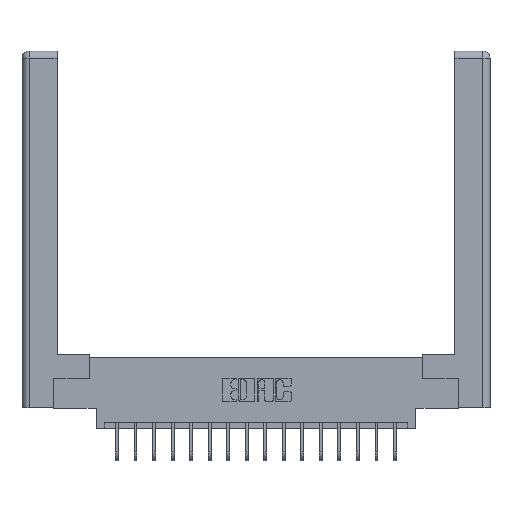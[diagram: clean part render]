
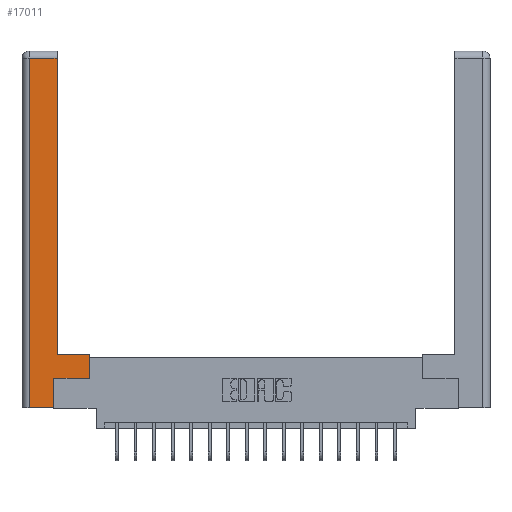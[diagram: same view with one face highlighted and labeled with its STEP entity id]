
A CAD part, top view. The second image highlights one B-rep face of the part: STEP entity #17011.
In plain terms, the highlighted planar face has unit normal (0, 0, 1).
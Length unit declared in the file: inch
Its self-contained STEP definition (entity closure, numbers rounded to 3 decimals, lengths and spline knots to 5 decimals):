
#185 = CARTESIAN_POINT ( 'NONE',  ( 0.265, 0.245, 0. ) ) ;
#501 = EDGE_CURVE ( 'NONE', #12441, #10015, #13441, .T. ) ;
#555 = VERTEX_POINT ( 'NONE', #2148 ) ;
#825 = LINE ( 'NONE', #7558, #19997 ) ;
#933 = CARTESIAN_POINT ( 'NONE',  ( 0.265, 0.245, 0. ) ) ;
#1471 = LINE ( 'NONE', #16307, #1960 ) ;
#1728 = CARTESIAN_POINT ( 'NONE',  ( 0.565, 0.245, 0. ) ) ;
#1729 = ORIENTED_EDGE ( 'NONE', *, *, #9157, .T. ) ;
#1960 = VECTOR ( 'NONE', #11657, 39.37008 ) ;
#2148 = CARTESIAN_POINT ( 'NONE',  ( 0.565, 0.245, 0. ) ) ;
#2303 = EDGE_LOOP ( 'NONE', ( #12869, #15334, #15696, #9023, #11551, #5707, #1729, #14557 ) ) ;
#2415 = PLANE ( 'NONE',  #19945 ) ;
#2545 = VECTOR ( 'NONE', #11239, 39.37008 ) ;
#3287 = CARTESIAN_POINT ( 'NONE',  ( 0.0615, 2.94, 0. ) ) ;
#4849 = DIRECTION ( 'NONE',  ( -1., 0., 0. ) ) ;
#4950 = CARTESIAN_POINT ( 'NONE',  ( 0.295, 2.94, 0. ) ) ;
#5299 = CARTESIAN_POINT ( 'NONE',  ( 0., 0., 0. ) ) ;
#5707 = ORIENTED_EDGE ( 'NONE', *, *, #6913, .T. ) ;
#6329 = EDGE_CURVE ( 'NONE', #10642, #17153, #825, .T. ) ;
#6685 = DIRECTION ( 'NONE',  ( -1., 0., 0. ) ) ;
#6752 = LINE ( 'NONE', #1728, #2545 ) ;
#6913 = EDGE_CURVE ( 'NONE', #12769, #555, #6752, .T. ) ;
#7241 = DIRECTION ( 'NONE',  ( -1., 0., 0. ) ) ;
#7310 = LINE ( 'NONE', #19363, #11980 ) ;
#7325 = VECTOR ( 'NONE', #4849, 39.37008 ) ;
#7428 = EDGE_CURVE ( 'NONE', #17153, #12769, #11880, .T. ) ;
#7558 = CARTESIAN_POINT ( 'NONE',  ( 0.265, 0., 0. ) ) ;
#8704 = VECTOR ( 'NONE', #11945, 39.37008 ) ;
#8774 = DIRECTION ( 'NONE',  ( 0., 0., -1. ) ) ;
#8837 = EDGE_CURVE ( 'NONE', #10015, #18423, #1471, .T. ) ;
#9023 = ORIENTED_EDGE ( 'NONE', *, *, #6329, .T. ) ;
#9157 = EDGE_CURVE ( 'NONE', #555, #12441, #19403, .T. ) ;
#9784 = VERTEX_POINT ( 'NONE', #3287 ) ;
#9792 = EDGE_CURVE ( 'NONE', #18423, #9784, #9849, .T. ) ;
#9849 = LINE ( 'NONE', #18941, #7325 ) ;
#10015 = VERTEX_POINT ( 'NONE', #18002 ) ;
#10030 = CARTESIAN_POINT ( 'NONE',  ( 0.0615, 0., 0. ) ) ;
#10642 = VERTEX_POINT ( 'NONE', #10030 ) ;
#10835 = FACE_OUTER_BOUND ( 'NONE', #2303, .T. ) ;
#11089 = VECTOR ( 'NONE', #17336, 39.37008 ) ;
#11239 = DIRECTION ( 'NONE',  ( 1., 0., 0. ) ) ;
#11551 = ORIENTED_EDGE ( 'NONE', *, *, #7428, .T. ) ;
#11657 = DIRECTION ( 'NONE',  ( 0., 1., 0. ) ) ;
#11724 = EDGE_CURVE ( 'NONE', #9784, #10642, #7310, .T. ) ;
#11880 = LINE ( 'NONE', #933, #8704 ) ;
#11945 = DIRECTION ( 'NONE',  ( 0., 1., 0. ) ) ;
#11976 = VECTOR ( 'NONE', #6685, 39.37008 ) ;
#11980 = VECTOR ( 'NONE', #14733, 39.37008 ) ;
#12441 = VERTEX_POINT ( 'NONE', #13659 ) ;
#12769 = VERTEX_POINT ( 'NONE', #185 ) ;
#12869 = ORIENTED_EDGE ( 'NONE', *, *, #8837, .T. ) ;
#13441 = LINE ( 'NONE', #17613, #11976 ) ;
#13659 = CARTESIAN_POINT ( 'NONE',  ( 0.565, 0.45, 0. ) ) ;
#14557 = ORIENTED_EDGE ( 'NONE', *, *, #501, .T. ) ;
#14733 = DIRECTION ( 'NONE',  ( 0., -1., 0. ) ) ;
#15334 = ORIENTED_EDGE ( 'NONE', *, *, #9792, .T. ) ;
#15696 = ORIENTED_EDGE ( 'NONE', *, *, #11724, .T. ) ;
#16307 = CARTESIAN_POINT ( 'NONE',  ( 0.295, 3., 0. ) ) ;
#17011 = ADVANCED_FACE ( 'NONE', ( #10835 ), #2415, .F. ) ;
#17153 = VERTEX_POINT ( 'NONE', #17386 ) ;
#17336 = DIRECTION ( 'NONE',  ( 0., 1., 0. ) ) ;
#17386 = CARTESIAN_POINT ( 'NONE',  ( 0.265, 0., 0. ) ) ;
#17613 = CARTESIAN_POINT ( 'NONE',  ( 0.295, 0.45, 0. ) ) ;
#18002 = CARTESIAN_POINT ( 'NONE',  ( 0.295, 0.45, 0. ) ) ;
#18423 = VERTEX_POINT ( 'NONE', #4950 ) ;
#18758 = CARTESIAN_POINT ( 'NONE',  ( 0.565, 0.45, 0. ) ) ;
#18941 = CARTESIAN_POINT ( 'NONE',  ( 0.0615, 2.94, 0. ) ) ;
#19363 = CARTESIAN_POINT ( 'NONE',  ( 0.0615, 0., 0. ) ) ;
#19403 = LINE ( 'NONE', #18758, #11089 ) ;
#19945 = AXIS2_PLACEMENT_3D ( 'NONE', #5299, #8774, #7241 ) ;
#19997 = VECTOR ( 'NONE', #20158, 39.37008 ) ;
#20158 = DIRECTION ( 'NONE',  ( 1., 0., 0. ) ) ;
